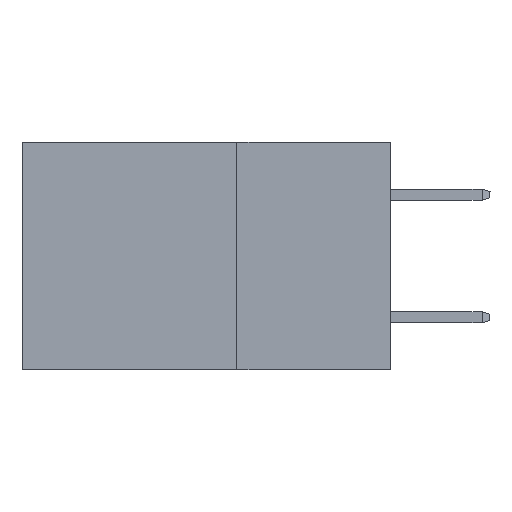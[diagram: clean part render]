
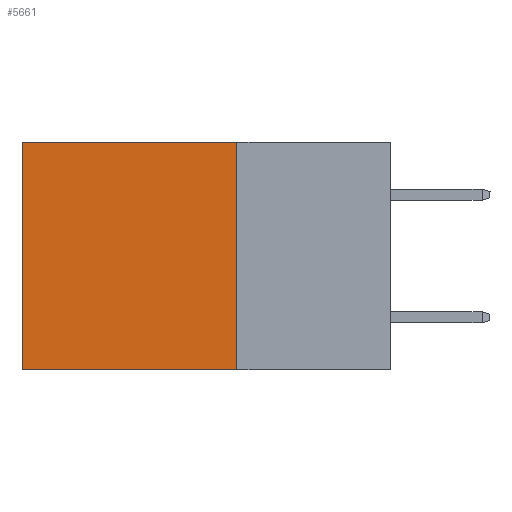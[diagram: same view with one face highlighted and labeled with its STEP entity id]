
A CAD part, left-side view. The second image highlights one B-rep face of the part: STEP entity #5661.
In plain terms, the highlighted planar face has unit normal (-1, 0, 0).
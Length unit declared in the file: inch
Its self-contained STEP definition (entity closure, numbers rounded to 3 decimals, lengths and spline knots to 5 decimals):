
#401 = ORIENTED_EDGE ( 'NONE', *, *, #995, .T. ) ;
#612 = EDGE_CURVE ( 'NONE', #2271, #13812, #18873, .T. ) ;
#972 = ORIENTED_EDGE ( 'NONE', *, *, #14277, .F. ) ;
#995 = EDGE_CURVE ( 'NONE', #1594, #13812, #17280, .T. ) ;
#1594 = VERTEX_POINT ( 'NONE', #3822 ) ;
#1982 = EDGE_LOOP ( 'NONE', ( #401, #2790, #972, #3246 ) ) ;
#2271 = VERTEX_POINT ( 'NONE', #15585 ) ;
#2637 = VECTOR ( 'NONE', #15949, 39.37008 ) ;
#2790 = ORIENTED_EDGE ( 'NONE', *, *, #612, .F. ) ;
#3072 = DIRECTION ( 'NONE',  ( 0., 0., -1. ) ) ;
#3246 = ORIENTED_EDGE ( 'NONE', *, *, #8462, .T. ) ;
#3731 = DIRECTION ( 'NONE',  ( 0., 1., 0. ) ) ;
#3822 = CARTESIAN_POINT ( 'NONE',  ( 0.2875, 0.6, 0. ) ) ;
#4131 = CARTESIAN_POINT ( 'NONE',  ( 0.2875, 0.25, 0. ) ) ;
#4202 = FACE_OUTER_BOUND ( 'NONE', #1982, .T. ) ;
#4673 = DIRECTION ( 'NONE',  ( 0., 0., -1. ) ) ;
#4684 = VECTOR ( 'NONE', #3072, 39.37008 ) ;
#4912 = CARTESIAN_POINT ( 'NONE',  ( 0.2875, 0.6, 0. ) ) ;
#5661 = ADVANCED_FACE ( 'NONE', ( #4202 ), #15767, .F. ) ;
#6693 = LINE ( 'NONE', #18818, #2637 ) ;
#7810 = CARTESIAN_POINT ( 'NONE',  ( 0.2875, 0.25, -0.37 ) ) ;
#7821 = VERTEX_POINT ( 'NONE', #4131 ) ;
#8462 = EDGE_CURVE ( 'NONE', #7821, #1594, #6693, .T. ) ;
#9247 = LINE ( 'NONE', #19328, #4684 ) ;
#13812 = VERTEX_POINT ( 'NONE', #16819 ) ;
#14277 = EDGE_CURVE ( 'NONE', #7821, #2271, #9247, .T. ) ;
#15477 = VECTOR ( 'NONE', #3731, 39.37008 ) ;
#15585 = CARTESIAN_POINT ( 'NONE',  ( 0.2875, 0.25, -0.37 ) ) ;
#15651 = DIRECTION ( 'NONE',  ( 0., 0., -1. ) ) ;
#15672 = DIRECTION ( 'NONE',  ( 1., 0., 0. ) ) ;
#15767 = PLANE ( 'NONE',  #18202 ) ;
#15940 = CARTESIAN_POINT ( 'NONE',  ( 0.2875, 0.25, 0. ) ) ;
#15949 = DIRECTION ( 'NONE',  ( 0., 1., 0. ) ) ;
#16819 = CARTESIAN_POINT ( 'NONE',  ( 0.2875, 0.6, -0.37 ) ) ;
#17280 = LINE ( 'NONE', #4912, #18192 ) ;
#18192 = VECTOR ( 'NONE', #4673, 39.37008 ) ;
#18202 = AXIS2_PLACEMENT_3D ( 'NONE', #15940, #15672, #15651 ) ;
#18818 = CARTESIAN_POINT ( 'NONE',  ( 0.2875, 0.25, 0. ) ) ;
#18873 = LINE ( 'NONE', #7810, #15477 ) ;
#19328 = CARTESIAN_POINT ( 'NONE',  ( 0.2875, 0.25, 0. ) ) ;
